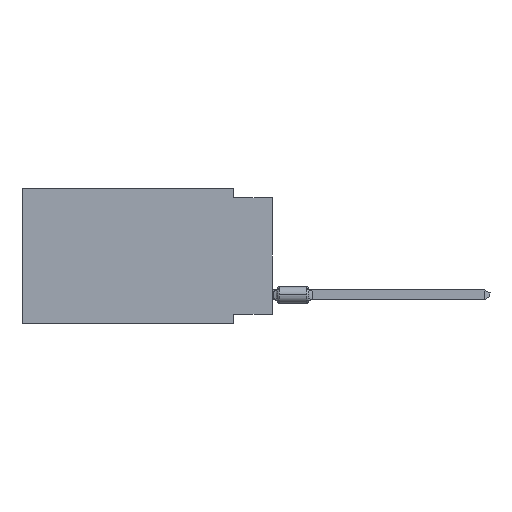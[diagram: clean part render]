
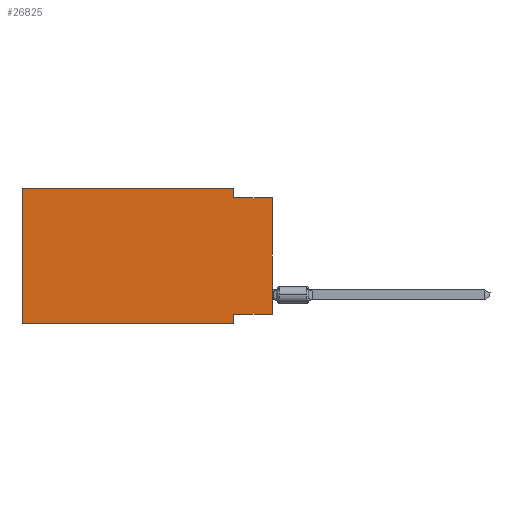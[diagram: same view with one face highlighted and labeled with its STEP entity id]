
A CAD part, left-side view. The second image highlights one B-rep face of the part: STEP entity #26825.
In plain terms, the highlighted planar face has unit normal (-1, 0, 0).
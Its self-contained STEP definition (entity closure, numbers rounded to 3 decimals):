
#944 = VERTEX_POINT ( 'NONE', #63445 ) ;
#1219 = ORIENTED_EDGE ( 'NONE', *, *, #17750, .F. ) ;
#1368 = EDGE_CURVE ( 'NONE', #71624, #91345, #47252, .T. ) ;
#2154 = DIRECTION ( 'NONE',  ( 0., -1., 0. ) ) ;
#2680 = LINE ( 'NONE', #39402, #81340 ) ;
#4762 = EDGE_CURVE ( 'NONE', #14064, #44956, #5034, .T. ) ;
#5034 = LINE ( 'NONE', #81453, #20976 ) ;
#6544 = EDGE_CURVE ( 'NONE', #60941, #14064, #23767, .T. ) ;
#9391 = DIRECTION ( 'NONE',  ( 0., 0., -1. ) ) ;
#9588 = CARTESIAN_POINT ( 'NONE',  ( 0., 16.383, -8.89 ) ) ;
#10314 = VECTOR ( 'NONE', #93218, 1000. ) ;
#13117 = ORIENTED_EDGE ( 'NONE', *, *, #6544, .F. ) ;
#14064 = VERTEX_POINT ( 'NONE', #62021 ) ;
#15241 = ORIENTED_EDGE ( 'NONE', *, *, #95410, .T. ) ;
#15275 = DIRECTION ( 'NONE',  ( 0., -1., 0. ) ) ;
#16986 = CARTESIAN_POINT ( 'NONE',  ( 0., 16.383, 0. ) ) ;
#17556 = CARTESIAN_POINT ( 'NONE',  ( 0., 0., -8.255 ) ) ;
#17750 = EDGE_CURVE ( 'NONE', #91345, #83819, #54386, .T. ) ;
#18010 = VECTOR ( 'NONE', #84653, 1000. ) ;
#18122 = CARTESIAN_POINT ( 'NONE',  ( 0., 16.383, 0. ) ) ;
#20976 = VECTOR ( 'NONE', #36260, 1000. ) ;
#23330 = FACE_OUTER_BOUND ( 'NONE', #59377, .T. ) ;
#23767 = LINE ( 'NONE', #32676, #10314 ) ;
#26825 = ADVANCED_FACE ( 'NONE', ( #23330 ), #30768, .F. ) ;
#30643 = LINE ( 'NONE', #92149, #48318 ) ;
#30768 = PLANE ( 'NONE',  #81872 ) ;
#32676 = CARTESIAN_POINT ( 'NONE',  ( 0., 0., -8.255 ) ) ;
#36256 = EDGE_CURVE ( 'NONE', #83819, #944, #89752, .T. ) ;
#36260 = DIRECTION ( 'NONE',  ( 0., 0., -1. ) ) ;
#38421 = ORIENTED_EDGE ( 'NONE', *, *, #68184, .F. ) ;
#39402 = CARTESIAN_POINT ( 'NONE',  ( 0., 0., 0. ) ) ;
#43262 = CARTESIAN_POINT ( 'NONE',  ( 0., 16.383, -8.89 ) ) ;
#44956 = VERTEX_POINT ( 'NONE', #87368 ) ;
#47252 = LINE ( 'NONE', #16986, #76170 ) ;
#48318 = VECTOR ( 'NONE', #15275, 1000. ) ;
#51887 = CARTESIAN_POINT ( 'NONE',  ( 0., 16.383, 0. ) ) ;
#53237 = CARTESIAN_POINT ( 'NONE',  ( 0., 0., -0.635 ) ) ;
#54386 = LINE ( 'NONE', #18122, #18010 ) ;
#54387 = ORIENTED_EDGE ( 'NONE', *, *, #4762, .F. ) ;
#58512 = DIRECTION ( 'NONE',  ( 0., 0., -1. ) ) ;
#58660 = ORIENTED_EDGE ( 'NONE', *, *, #64496, .T. ) ;
#59377 = EDGE_LOOP ( 'NONE', ( #58660, #38421, #83557, #1219, #75374, #15241, #54387, #13117 ) ) ;
#59992 = CARTESIAN_POINT ( 'NONE',  ( 0., 2.54, 0. ) ) ;
#60941 = VERTEX_POINT ( 'NONE', #17556 ) ;
#61051 = DIRECTION ( 'NONE',  ( 1., 0., 0. ) ) ;
#61252 = LINE ( 'NONE', #9588, #69495 ) ;
#62021 = CARTESIAN_POINT ( 'NONE',  ( 0., 2.54, -8.255 ) ) ;
#63445 = CARTESIAN_POINT ( 'NONE',  ( 0., 2.54, -0.635 ) ) ;
#64496 = EDGE_CURVE ( 'NONE', #60941, #64880, #2680, .T. ) ;
#64880 = VERTEX_POINT ( 'NONE', #53237 ) ;
#68184 = EDGE_CURVE ( 'NONE', #944, #64880, #30643, .T. ) ;
#69495 = VECTOR ( 'NONE', #2154, 1000. ) ;
#71624 = VERTEX_POINT ( 'NONE', #43262 ) ;
#75374 = ORIENTED_EDGE ( 'NONE', *, *, #1368, .F. ) ;
#76170 = VECTOR ( 'NONE', #77507, 1000. ) ;
#77383 = CARTESIAN_POINT ( 'NONE',  ( 0., 16.383, 0. ) ) ;
#77507 = DIRECTION ( 'NONE',  ( 0., 0., 1. ) ) ;
#81340 = VECTOR ( 'NONE', #86531, 1000. ) ;
#81453 = CARTESIAN_POINT ( 'NONE',  ( 0., 2.54, -8.89 ) ) ;
#81872 = AXIS2_PLACEMENT_3D ( 'NONE', #77383, #61051, #9391 ) ;
#83557 = ORIENTED_EDGE ( 'NONE', *, *, #36256, .F. ) ;
#83819 = VERTEX_POINT ( 'NONE', #87335 ) ;
#84653 = DIRECTION ( 'NONE',  ( 0., -1., 0. ) ) ;
#86531 = DIRECTION ( 'NONE',  ( 0., 0., 1. ) ) ;
#87335 = CARTESIAN_POINT ( 'NONE',  ( 0., 2.54, 0. ) ) ;
#87368 = CARTESIAN_POINT ( 'NONE',  ( 0., 2.54, -8.89 ) ) ;
#87803 = VECTOR ( 'NONE', #58512, 1000. ) ;
#89752 = LINE ( 'NONE', #59992, #87803 ) ;
#91345 = VERTEX_POINT ( 'NONE', #51887 ) ;
#92149 = CARTESIAN_POINT ( 'NONE',  ( 0., 0., -0.635 ) ) ;
#93218 = DIRECTION ( 'NONE',  ( 0., 1., 0. ) ) ;
#95410 = EDGE_CURVE ( 'NONE', #71624, #44956, #61252, .T. ) ;
